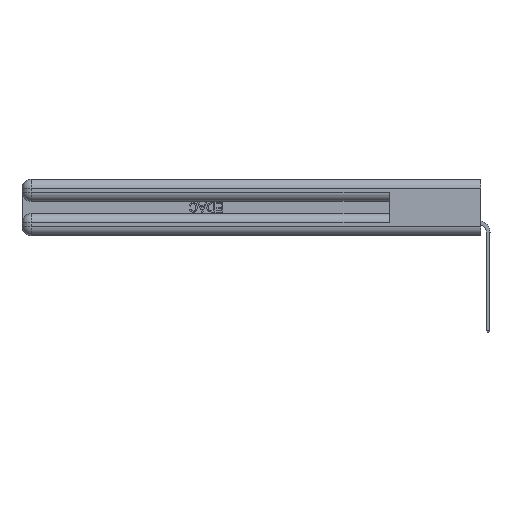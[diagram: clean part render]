
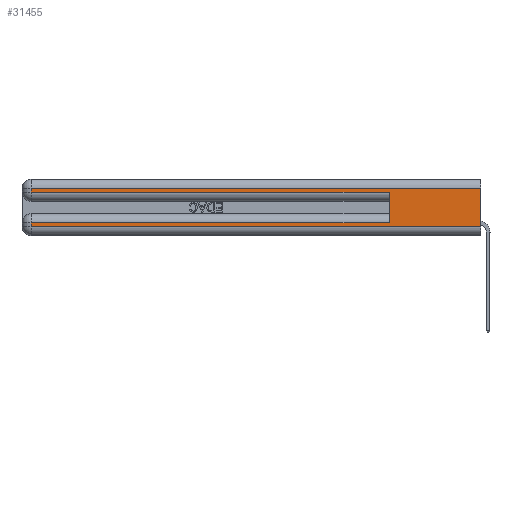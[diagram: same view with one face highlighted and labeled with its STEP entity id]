
A CAD part, left-side view. The second image highlights one B-rep face of the part: STEP entity #31455.
In plain terms, the highlighted planar face has unit normal (-1, 0, 0).
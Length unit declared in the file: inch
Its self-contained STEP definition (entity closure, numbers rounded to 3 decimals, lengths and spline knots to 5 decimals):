
#32 = ORIENTED_EDGE ( 'NONE', *, *, #7673, .T. ) ;
#430 = LINE ( 'NONE', #18731, #14596 ) ;
#1163 = DIRECTION ( 'NONE',  ( 0., 0., -1. ) ) ;
#1710 = VECTOR ( 'NONE', #25838, 39.37008 ) ;
#2518 = EDGE_CURVE ( 'NONE', #4554, #6321, #430, .T. ) ;
#4554 = VERTEX_POINT ( 'NONE', #13734 ) ;
#4619 = DIRECTION ( 'NONE',  ( 0., 1., 0. ) ) ;
#6317 = CARTESIAN_POINT ( 'NONE',  ( 0., 2.94, 0.085 ) ) ;
#6321 = VERTEX_POINT ( 'NONE', #46441 ) ;
#7673 = EDGE_CURVE ( 'NONE', #25559, #38095, #24571, .T. ) ;
#8538 = LINE ( 'NONE', #47472, #26396 ) ;
#11076 = CARTESIAN_POINT ( 'NONE',  ( 0., 2.94, 0.285 ) ) ;
#11270 = CARTESIAN_POINT ( 'NONE',  ( 0., 0., 0.285 ) ) ;
#12355 = CARTESIAN_POINT ( 'NONE',  ( 0., 0.6, 0.145 ) ) ;
#12817 = VECTOR ( 'NONE', #4619, 39.37008 ) ;
#13734 = CARTESIAN_POINT ( 'NONE',  ( 0., 0., 0.31 ) ) ;
#14161 = VECTOR ( 'NONE', #1163, 39.37008 ) ;
#14564 = LINE ( 'NONE', #12355, #44894 ) ;
#14596 = VECTOR ( 'NONE', #42826, 39.37008 ) ;
#14844 = EDGE_CURVE ( 'NONE', #38095, #28872, #16929, .T. ) ;
#15835 = DIRECTION ( 'NONE',  ( 0., 1., 0. ) ) ;
#15903 = VECTOR ( 'NONE', #33356, 39.37008 ) ;
#16623 = DIRECTION ( 'NONE',  ( 0., 0., -1. ) ) ;
#16673 = VERTEX_POINT ( 'NONE', #33936 ) ;
#16726 = ORIENTED_EDGE ( 'NONE', *, *, #48004, .F. ) ;
#16929 = LINE ( 'NONE', #11270, #44157 ) ;
#18355 = VERTEX_POINT ( 'NONE', #6317 ) ;
#18641 = EDGE_CURVE ( 'NONE', #43264, #18355, #8538, .T. ) ;
#18731 = CARTESIAN_POINT ( 'NONE',  ( 0., 0., 0.37 ) ) ;
#21518 = CARTESIAN_POINT ( 'NONE',  ( 0., 0., 0.06 ) ) ;
#22558 = EDGE_LOOP ( 'NONE', ( #34146, #41307, #32, #22801, #16726, #31999, #46287, #29063 ) ) ;
#22801 = ORIENTED_EDGE ( 'NONE', *, *, #14844, .T. ) ;
#24571 = LINE ( 'NONE', #40334, #14161 ) ;
#25559 = VERTEX_POINT ( 'NONE', #35430 ) ;
#25838 = DIRECTION ( 'NONE',  ( 0., -1., 0. ) ) ;
#26396 = VECTOR ( 'NONE', #15835, 39.37008 ) ;
#27694 = DIRECTION ( 'NONE',  ( 0., 0., 1. ) ) ;
#28186 = CARTESIAN_POINT ( 'NONE',  ( 0., 0., 0.31 ) ) ;
#28872 = VERTEX_POINT ( 'NONE', #35588 ) ;
#29063 = ORIENTED_EDGE ( 'NONE', *, *, #35859, .T. ) ;
#29691 = PLANE ( 'NONE',  #41214 ) ;
#31455 = ADVANCED_FACE ( 'NONE', ( #32961 ), #29691, .F. ) ;
#31972 = LINE ( 'NONE', #28186, #12817 ) ;
#31999 = ORIENTED_EDGE ( 'NONE', *, *, #18641, .T. ) ;
#32961 = FACE_OUTER_BOUND ( 'NONE', #22558, .T. ) ;
#33356 = DIRECTION ( 'NONE',  ( 0., 0., -1. ) ) ;
#33936 = CARTESIAN_POINT ( 'NONE',  ( 0., 2.94, 0.06 ) ) ;
#34146 = ORIENTED_EDGE ( 'NONE', *, *, #2518, .F. ) ;
#35176 = EDGE_CURVE ( 'NONE', #4554, #25559, #31972, .T. ) ;
#35430 = CARTESIAN_POINT ( 'NONE',  ( 0., 2.94, 0.31 ) ) ;
#35588 = CARTESIAN_POINT ( 'NONE',  ( 0., 0.6, 0.285 ) ) ;
#35859 = EDGE_CURVE ( 'NONE', #16673, #6321, #38146, .T. ) ;
#37686 = DIRECTION ( 'NONE',  ( 0., -1., 0. ) ) ;
#38095 = VERTEX_POINT ( 'NONE', #11076 ) ;
#38146 = LINE ( 'NONE', #21518, #1710 ) ;
#40334 = CARTESIAN_POINT ( 'NONE',  ( 0., 2.94, 0.37 ) ) ;
#41214 = AXIS2_PLACEMENT_3D ( 'NONE', #46821, #47420, #16623 ) ;
#41307 = ORIENTED_EDGE ( 'NONE', *, *, #35176, .T. ) ;
#42826 = DIRECTION ( 'NONE',  ( 0., 0., -1. ) ) ;
#43264 = VERTEX_POINT ( 'NONE', #48655 ) ;
#44157 = VECTOR ( 'NONE', #37686, 39.37008 ) ;
#44894 = VECTOR ( 'NONE', #27694, 39.37008 ) ;
#45298 = CARTESIAN_POINT ( 'NONE',  ( 0., 2.94, 0.37 ) ) ;
#46287 = ORIENTED_EDGE ( 'NONE', *, *, #46983, .T. ) ;
#46441 = CARTESIAN_POINT ( 'NONE',  ( 0., 0., 0.06 ) ) ;
#46821 = CARTESIAN_POINT ( 'NONE',  ( 0., 0., 0.37 ) ) ;
#46884 = LINE ( 'NONE', #45298, #15903 ) ;
#46983 = EDGE_CURVE ( 'NONE', #18355, #16673, #46884, .T. ) ;
#47420 = DIRECTION ( 'NONE',  ( 1., 0., 0. ) ) ;
#47472 = CARTESIAN_POINT ( 'NONE',  ( 0., 0., 0.085 ) ) ;
#48004 = EDGE_CURVE ( 'NONE', #43264, #28872, #14564, .T. ) ;
#48655 = CARTESIAN_POINT ( 'NONE',  ( 0., 0.6, 0.085 ) ) ;
